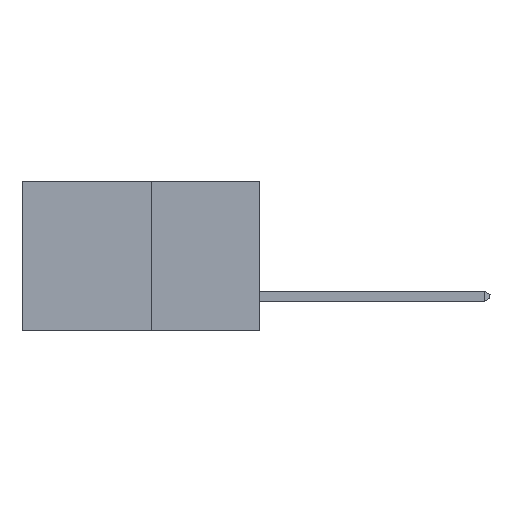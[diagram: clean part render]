
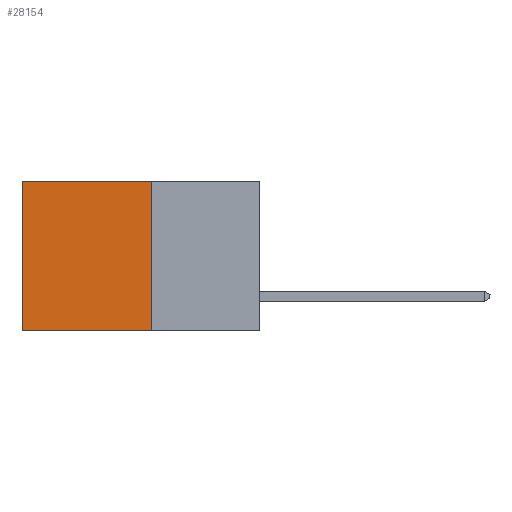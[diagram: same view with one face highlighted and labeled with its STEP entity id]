
A CAD part, left-side view. The second image highlights one B-rep face of the part: STEP entity #28154.
In plain terms, the highlighted planar face has unit normal (-1, 0, 0).
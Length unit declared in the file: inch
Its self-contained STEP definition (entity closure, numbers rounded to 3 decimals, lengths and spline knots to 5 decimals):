
#1369 = VECTOR ( 'NONE', #7113, 39.37008 ) ;
#1900 = CARTESIAN_POINT ( 'NONE',  ( 0.277, 0.59, 0. ) ) ;
#2957 = LINE ( 'NONE', #15127, #3637 ) ;
#3308 = EDGE_CURVE ( 'NONE', #10299, #18373, #18336, .T. ) ;
#3461 = EDGE_CURVE ( 'NONE', #10299, #23241, #14103, .T. ) ;
#3637 = VECTOR ( 'NONE', #6330, 39.37008 ) ;
#3921 = PLANE ( 'NONE',  #7151 ) ;
#6330 = DIRECTION ( 'NONE',  ( 0., 0., -1. ) ) ;
#6618 = FACE_OUTER_BOUND ( 'NONE', #19571, .T. ) ;
#7113 = DIRECTION ( 'NONE',  ( 0., 1., 0. ) ) ;
#7151 = AXIS2_PLACEMENT_3D ( 'NONE', #8384, #24009, #10645 ) ;
#8384 = CARTESIAN_POINT ( 'NONE',  ( 0.277, 0.27, -0.37 ) ) ;
#8509 = CARTESIAN_POINT ( 'NONE',  ( 0.277, 0.27, -0.37 ) ) ;
#8523 = EDGE_CURVE ( 'NONE', #23241, #11237, #25121, .T. ) ;
#8691 = DIRECTION ( 'NONE',  ( 0., 0., -1. ) ) ;
#10299 = VERTEX_POINT ( 'NONE', #12117 ) ;
#10645 = DIRECTION ( 'NONE',  ( 0., 0., -1. ) ) ;
#11075 = CARTESIAN_POINT ( 'NONE',  ( 0.277, 0.27, -0.37 ) ) ;
#11237 = VERTEX_POINT ( 'NONE', #15156 ) ;
#12117 = CARTESIAN_POINT ( 'NONE',  ( 0.277, 0.27, 0. ) ) ;
#12430 = VECTOR ( 'NONE', #28953, 39.37008 ) ;
#14103 = LINE ( 'NONE', #8509, #26094 ) ;
#15127 = CARTESIAN_POINT ( 'NONE',  ( 0.277, 0.59, -0.37 ) ) ;
#15156 = CARTESIAN_POINT ( 'NONE',  ( 0.277, 0.59, -0.37 ) ) ;
#15941 = CARTESIAN_POINT ( 'NONE',  ( 0.277, 0.27, -0.37 ) ) ;
#17402 = CARTESIAN_POINT ( 'NONE',  ( 0.277, 0.27, 0. ) ) ;
#18336 = LINE ( 'NONE', #17402, #12430 ) ;
#18373 = VERTEX_POINT ( 'NONE', #1900 ) ;
#18376 = EDGE_CURVE ( 'NONE', #18373, #11237, #2957, .T. ) ;
#18649 = ORIENTED_EDGE ( 'NONE', *, *, #3461, .F. ) ;
#19571 = EDGE_LOOP ( 'NONE', ( #23353, #27476, #18649, #21447 ) ) ;
#21447 = ORIENTED_EDGE ( 'NONE', *, *, #3308, .T. ) ;
#23241 = VERTEX_POINT ( 'NONE', #11075 ) ;
#23353 = ORIENTED_EDGE ( 'NONE', *, *, #18376, .T. ) ;
#24009 = DIRECTION ( 'NONE',  ( 1., 0., 0. ) ) ;
#25121 = LINE ( 'NONE', #15941, #1369 ) ;
#26094 = VECTOR ( 'NONE', #8691, 39.37008 ) ;
#27476 = ORIENTED_EDGE ( 'NONE', *, *, #8523, .F. ) ;
#28154 = ADVANCED_FACE ( 'NONE', ( #6618 ), #3921, .F. ) ;
#28953 = DIRECTION ( 'NONE',  ( 0., 1., 0. ) ) ;
